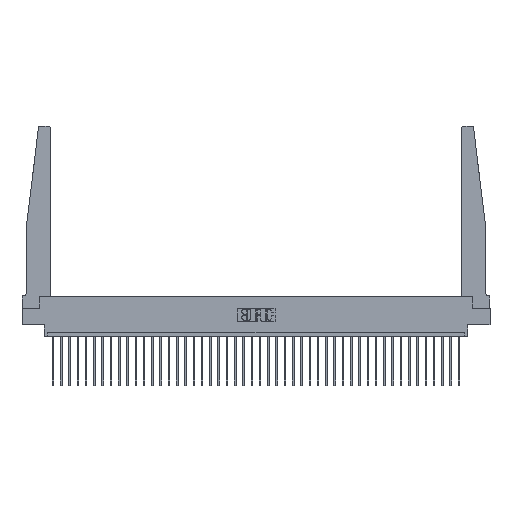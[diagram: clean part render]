
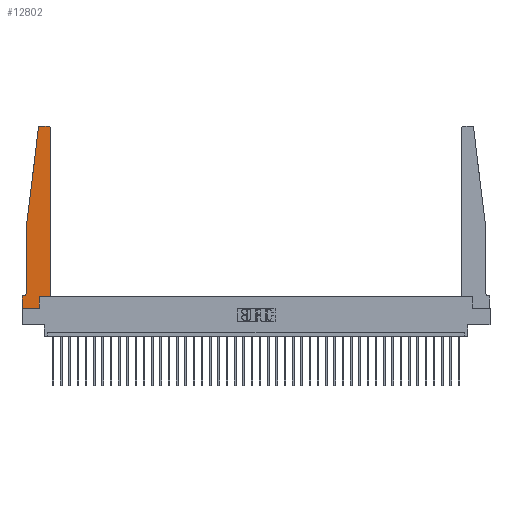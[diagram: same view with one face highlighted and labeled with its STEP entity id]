
A CAD part, top view. The second image highlights one B-rep face of the part: STEP entity #12802.
In plain terms, the highlighted planar face has unit normal (0, 0, 1).
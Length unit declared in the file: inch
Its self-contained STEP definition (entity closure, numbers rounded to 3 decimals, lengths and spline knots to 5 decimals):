
#272 = LINE ( 'NONE', #32769, #13616 ) ;
#389 = DIRECTION ( 'NONE',  ( -1., 0., 0. ) ) ;
#578 = AXIS2_PLACEMENT_3D ( 'NONE', #30448, #19211, #3279 ) ;
#1084 = EDGE_CURVE ( 'NONE', #14864, #32939, #31731, .T. ) ;
#1803 = DIRECTION ( 'NONE',  ( 0., 0., 1. ) ) ;
#1869 = LINE ( 'NONE', #31326, #8241 ) ;
#2089 = CARTESIAN_POINT ( 'NONE',  ( 0.425, 0.18, 0.37 ) ) ;
#2479 = VERTEX_POINT ( 'NONE', #21921 ) ;
#2907 = VERTEX_POINT ( 'NONE', #5891 ) ;
#3279 = DIRECTION ( 'NONE',  ( -1., 0., 0. ) ) ;
#4477 = PLANE ( 'NONE',  #23554 ) ;
#4731 = EDGE_LOOP ( 'NONE', ( #28762, #34210, #25784, #21892, #16145, #16719, #32203, #26510, #23134, #12892, #20889, #7402 ) ) ;
#5001 = CARTESIAN_POINT ( 'NONE',  ( 0., 0.1875, 0.37 ) ) ;
#5891 = CARTESIAN_POINT ( 'NONE',  ( 0.015, 0.1875, 0.37 ) ) ;
#5895 = CARTESIAN_POINT ( 'NONE',  ( 0.27653, 2.72, 0.37 ) ) ;
#6508 = EDGE_CURVE ( 'NONE', #14126, #2479, #272, .T. ) ;
#6931 = DIRECTION ( 'NONE',  ( 0., 1., 0. ) ) ;
#7273 = DIRECTION ( 'NONE',  ( 0., 1., 0. ) ) ;
#7277 = LINE ( 'NONE', #18174, #26536 ) ;
#7402 = ORIENTED_EDGE ( 'NONE', *, *, #27825, .T. ) ;
#8241 = VECTOR ( 'NONE', #17595, 39.37008 ) ;
#8425 = CARTESIAN_POINT ( 'NONE',  ( 0.065, 0.1875, 0.37 ) ) ;
#8537 = VECTOR ( 'NONE', #13307, 39.37008 ) ;
#8654 = VERTEX_POINT ( 'NONE', #18962 ) ;
#9823 = DIRECTION ( 'NONE',  ( 1., 0., 0. ) ) ;
#10220 = CARTESIAN_POINT ( 'NONE',  ( 0.425, 0.18, 0.37 ) ) ;
#10370 = VERTEX_POINT ( 'NONE', #30171 ) ;
#11148 = CARTESIAN_POINT ( 'NONE',  ( 0.425, 2.72, 0.37 ) ) ;
#12365 = VERTEX_POINT ( 'NONE', #32009 ) ;
#12501 = EDGE_CURVE ( 'NONE', #2907, #32367, #32888, .T. ) ;
#12802 = ADVANCED_FACE ( 'NONE', ( #23403 ), #4477, .T. ) ;
#12892 = ORIENTED_EDGE ( 'NONE', *, *, #33215, .T. ) ;
#13307 = DIRECTION ( 'NONE',  ( -1., 0., 0. ) ) ;
#13616 = VECTOR ( 'NONE', #22060, 39.37008 ) ;
#14126 = VERTEX_POINT ( 'NONE', #32673 ) ;
#14498 = VERTEX_POINT ( 'NONE', #24431 ) ;
#14864 = VERTEX_POINT ( 'NONE', #21864 ) ;
#15999 = VECTOR ( 'NONE', #20955, 39.37008 ) ;
#16001 = CIRCLE ( 'NONE', #578, 0.05 ) ;
#16145 = ORIENTED_EDGE ( 'NONE', *, *, #18764, .T. ) ;
#16719 = ORIENTED_EDGE ( 'NONE', *, *, #12501, .T. ) ;
#17481 = LINE ( 'NONE', #28372, #27952 ) ;
#17595 = DIRECTION ( 'NONE',  ( -0.122, -0.992, 0. ) ) ;
#17612 = DIRECTION ( 'NONE',  ( 1., 0., 0. ) ) ;
#18174 = CARTESIAN_POINT ( 'NONE',  ( 0.2605, 0.18, 0.37 ) ) ;
#18564 = AXIS2_PLACEMENT_3D ( 'NONE', #33665, #19757, #17612 ) ;
#18764 = EDGE_CURVE ( 'NONE', #14498, #2907, #16001, .T. ) ;
#18962 = CARTESIAN_POINT ( 'NONE',  ( 0.24675, 2.72367, 0.37 ) ) ;
#19211 = DIRECTION ( 'NONE',  ( 0., 0., -1. ) ) ;
#19457 = AXIS2_PLACEMENT_3D ( 'NONE', #5895, #33187, #32480 ) ;
#19757 = DIRECTION ( 'NONE',  ( 0., 0., 1. ) ) ;
#20019 = CIRCLE ( 'NONE', #19457, 0.03 ) ;
#20253 = CARTESIAN_POINT ( 'NONE',  ( 0.395, 2.75, 0.37 ) ) ;
#20889 = ORIENTED_EDGE ( 'NONE', *, *, #1084, .T. ) ;
#20955 = DIRECTION ( 'NONE',  ( 1., 0., 0. ) ) ;
#20992 = CARTESIAN_POINT ( 'NONE',  ( 0.25, 2.75, 0.37 ) ) ;
#21539 = VERTEX_POINT ( 'NONE', #20253 ) ;
#21864 = CARTESIAN_POINT ( 'NONE',  ( 0.425, 0.18, 0.37 ) ) ;
#21892 = ORIENTED_EDGE ( 'NONE', *, *, #32658, .T. ) ;
#21921 = CARTESIAN_POINT ( 'NONE',  ( 0.2605, 0., 0.37 ) ) ;
#22060 = DIRECTION ( 'NONE',  ( 1., 0., 0. ) ) ;
#22365 = VECTOR ( 'NONE', #389, 39.37008 ) ;
#22968 = VECTOR ( 'NONE', #7273, 39.37008 ) ;
#23134 = ORIENTED_EDGE ( 'NONE', *, *, #27551, .T. ) ;
#23403 = FACE_OUTER_BOUND ( 'NONE', #4731, .T. ) ;
#23554 = AXIS2_PLACEMENT_3D ( 'NONE', #34287, #1803, #9823 ) ;
#24047 = LINE ( 'NONE', #34934, #24849 ) ;
#24277 = VERTEX_POINT ( 'NONE', #32640 ) ;
#24431 = CARTESIAN_POINT ( 'NONE',  ( 0.065, 0.2375, 0.37 ) ) ;
#24582 = DIRECTION ( 'NONE',  ( 0., -1., 0. ) ) ;
#24849 = VECTOR ( 'NONE', #24582, 39.37008 ) ;
#24944 = EDGE_CURVE ( 'NONE', #8654, #10370, #1869, .T. ) ;
#25687 = DIRECTION ( 'NONE',  ( 0., -1., 0. ) ) ;
#25784 = ORIENTED_EDGE ( 'NONE', *, *, #24944, .T. ) ;
#25911 = EDGE_CURVE ( 'NONE', #32367, #14126, #24047, .T. ) ;
#26510 = ORIENTED_EDGE ( 'NONE', *, *, #6508, .T. ) ;
#26536 = VECTOR ( 'NONE', #6931, 39.37008 ) ;
#27551 = EDGE_CURVE ( 'NONE', #2479, #24277, #7277, .T. ) ;
#27825 = EDGE_CURVE ( 'NONE', #32939, #21539, #29416, .T. ) ;
#27952 = VECTOR ( 'NONE', #25687, 39.37008 ) ;
#28372 = CARTESIAN_POINT ( 'NONE',  ( 0.065, 1.25, 0.37 ) ) ;
#28762 = ORIENTED_EDGE ( 'NONE', *, *, #32866, .T. ) ;
#29416 = CIRCLE ( 'NONE', #18564, 0.03 ) ;
#30171 = CARTESIAN_POINT ( 'NONE',  ( 0.065, 1.25, 0.37 ) ) ;
#30448 = CARTESIAN_POINT ( 'NONE',  ( 0.015, 0.2375, 0.37 ) ) ;
#31326 = CARTESIAN_POINT ( 'NONE',  ( 0.065, 1.25, 0.37 ) ) ;
#31731 = LINE ( 'NONE', #2089, #22968 ) ;
#32009 = CARTESIAN_POINT ( 'NONE',  ( 0.27653, 2.75, 0.37 ) ) ;
#32203 = ORIENTED_EDGE ( 'NONE', *, *, #25911, .T. ) ;
#32367 = VERTEX_POINT ( 'NONE', #5001 ) ;
#32480 = DIRECTION ( 'NONE',  ( 1., 0., 0. ) ) ;
#32640 = CARTESIAN_POINT ( 'NONE',  ( 0.2605, 0.18, 0.37 ) ) ;
#32658 = EDGE_CURVE ( 'NONE', #10370, #14498, #17481, .T. ) ;
#32673 = CARTESIAN_POINT ( 'NONE',  ( 0., 0., 0.37 ) ) ;
#32769 = CARTESIAN_POINT ( 'NONE',  ( 0., 0., 0.37 ) ) ;
#32866 = EDGE_CURVE ( 'NONE', #21539, #12365, #35251, .T. ) ;
#32888 = LINE ( 'NONE', #8425, #22365 ) ;
#32939 = VERTEX_POINT ( 'NONE', #11148 ) ;
#33187 = DIRECTION ( 'NONE',  ( 0., 0., 1. ) ) ;
#33215 = EDGE_CURVE ( 'NONE', #24277, #14864, #34324, .T. ) ;
#33665 = CARTESIAN_POINT ( 'NONE',  ( 0.395, 2.72, 0.37 ) ) ;
#33834 = EDGE_CURVE ( 'NONE', #12365, #8654, #20019, .T. ) ;
#34210 = ORIENTED_EDGE ( 'NONE', *, *, #33834, .T. ) ;
#34287 = CARTESIAN_POINT ( 'NONE',  ( 0., 0.1875, 0.37 ) ) ;
#34324 = LINE ( 'NONE', #10220, #15999 ) ;
#34934 = CARTESIAN_POINT ( 'NONE',  ( 0., 0., 0.37 ) ) ;
#35251 = LINE ( 'NONE', #20992, #8537 ) ;
